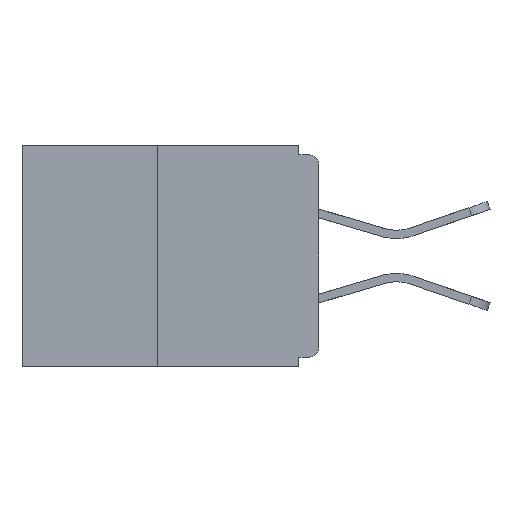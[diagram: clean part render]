
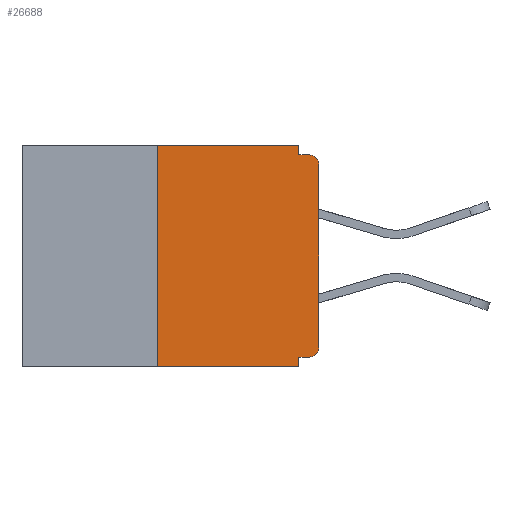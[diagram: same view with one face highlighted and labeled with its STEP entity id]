
A CAD part, left-side view. The second image highlights one B-rep face of the part: STEP entity #26688.
In plain terms, the highlighted planar face has unit normal (-1, 0, 0).
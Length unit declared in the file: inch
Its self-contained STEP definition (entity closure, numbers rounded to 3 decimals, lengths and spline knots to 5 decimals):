
#182 = CARTESIAN_POINT ( 'NONE',  ( 0., 0.031, 0. ) ) ;
#432 = CARTESIAN_POINT ( 'NONE',  ( 0., 0., -0.03 ) ) ;
#718 = VECTOR ( 'NONE', #28998, 39.37008 ) ;
#874 = CARTESIAN_POINT ( 'NONE',  ( 0., 0.031, -0.343 ) ) ;
#924 = DIRECTION ( 'NONE',  ( 1., 0., 0. ) ) ;
#1864 = VERTEX_POINT ( 'NONE', #21137 ) ;
#2328 = ORIENTED_EDGE ( 'NONE', *, *, #19186, .T. ) ;
#2341 = EDGE_CURVE ( 'NONE', #22695, #10764, #21661, .T. ) ;
#2389 = EDGE_LOOP ( 'NONE', ( #16454, #28490, #7199, #27091, #4894, #2328, #24212, #11146, #4104, #2781 ) ) ;
#2548 = DIRECTION ( 'NONE',  ( 0., -1., 0. ) ) ;
#2781 = ORIENTED_EDGE ( 'NONE', *, *, #2341, .F. ) ;
#2846 = CARTESIAN_POINT ( 'NONE',  ( 0., 0., -0.328 ) ) ;
#2960 = EDGE_CURVE ( 'NONE', #22089, #11140, #11749, .T. ) ;
#3183 = DIRECTION ( 'NONE',  ( 0., 0., -1. ) ) ;
#3487 = LINE ( 'NONE', #2846, #718 ) ;
#4104 = ORIENTED_EDGE ( 'NONE', *, *, #16299, .F. ) ;
#4231 = LINE ( 'NONE', #16019, #21391 ) ;
#4462 = AXIS2_PLACEMENT_3D ( 'NONE', #14657, #26265, #18916 ) ;
#4894 = ORIENTED_EDGE ( 'NONE', *, *, #9586, .F. ) ;
#6100 = DIRECTION ( 'NONE',  ( 0., 0., -1. ) ) ;
#6287 = CARTESIAN_POINT ( 'NONE',  ( 0., 0.46, 0. ) ) ;
#6521 = DIRECTION ( 'NONE',  ( 0., 0., 1. ) ) ;
#6545 = LINE ( 'NONE', #10493, #23635 ) ;
#6589 = CARTESIAN_POINT ( 'NONE',  ( 0., 0.46, -0.343 ) ) ;
#7199 = ORIENTED_EDGE ( 'NONE', *, *, #21327, .T. ) ;
#8883 = DIRECTION ( 'NONE',  ( 0., 0., -1. ) ) ;
#9586 = EDGE_CURVE ( 'NONE', #16956, #14985, #3487, .T. ) ;
#9768 = EDGE_CURVE ( 'NONE', #10097, #1864, #6545, .T. ) ;
#10097 = VERTEX_POINT ( 'NONE', #26069 ) ;
#10493 = CARTESIAN_POINT ( 'NONE',  ( 0., 0.25, 0. ) ) ;
#10764 = VERTEX_POINT ( 'NONE', #20231 ) ;
#11140 = VERTEX_POINT ( 'NONE', #432 ) ;
#11146 = ORIENTED_EDGE ( 'NONE', *, *, #27643, .T. ) ;
#11719 = VERTEX_POINT ( 'NONE', #24113 ) ;
#11749 = LINE ( 'NONE', #27129, #12750 ) ;
#11895 = LINE ( 'NONE', #25942, #18970 ) ;
#12056 = VERTEX_POINT ( 'NONE', #12471 ) ;
#12471 = CARTESIAN_POINT ( 'NONE',  ( 0., 0.015, -0.015 ) ) ;
#12750 = VECTOR ( 'NONE', #6521, 39.37008 ) ;
#13713 = AXIS2_PLACEMENT_3D ( 'NONE', #6287, #924, #15182 ) ;
#14065 = DIRECTION ( 'NONE',  ( 0., -1., 0. ) ) ;
#14657 = CARTESIAN_POINT ( 'NONE',  ( 0., 0.015, -0.03 ) ) ;
#14985 = VERTEX_POINT ( 'NONE', #28916 ) ;
#15182 = DIRECTION ( 'NONE',  ( 0., 0., -1. ) ) ;
#15641 = CARTESIAN_POINT ( 'NONE',  ( 0., 0.015, -0.328 ) ) ;
#16019 = CARTESIAN_POINT ( 'NONE',  ( 0., 0., -0.015 ) ) ;
#16299 = EDGE_CURVE ( 'NONE', #10764, #12056, #4231, .T. ) ;
#16454 = ORIENTED_EDGE ( 'NONE', *, *, #21848, .F. ) ;
#16956 = VERTEX_POINT ( 'NONE', #15641 ) ;
#17069 = VECTOR ( 'NONE', #6100, 39.37008 ) ;
#17446 = CARTESIAN_POINT ( 'NONE',  ( 0., 0.015, -0.313 ) ) ;
#18916 = DIRECTION ( 'NONE',  ( 0., 0., -1. ) ) ;
#18970 = VECTOR ( 'NONE', #2548, 39.37008 ) ;
#19078 = CIRCLE ( 'NONE', #4462, 0.015 ) ;
#19186 = EDGE_CURVE ( 'NONE', #16956, #22089, #26212, .T. ) ;
#19540 = LINE ( 'NONE', #874, #22490 ) ;
#20055 = FACE_OUTER_BOUND ( 'NONE', #2389, .T. ) ;
#20231 = CARTESIAN_POINT ( 'NONE',  ( 0., 0.031, -0.015 ) ) ;
#21137 = CARTESIAN_POINT ( 'NONE',  ( 0., 0.25, 0. ) ) ;
#21327 = EDGE_CURVE ( 'NONE', #10097, #11719, #29828, .T. ) ;
#21391 = VECTOR ( 'NONE', #22876, 39.37008 ) ;
#21661 = LINE ( 'NONE', #29165, #17069 ) ;
#21848 = EDGE_CURVE ( 'NONE', #1864, #22695, #11895, .T. ) ;
#22089 = VERTEX_POINT ( 'NONE', #30042 ) ;
#22490 = VECTOR ( 'NONE', #3183, 39.37008 ) ;
#22695 = VERTEX_POINT ( 'NONE', #182 ) ;
#22876 = DIRECTION ( 'NONE',  ( 0., -1., 0. ) ) ;
#23635 = VECTOR ( 'NONE', #29615, 39.37008 ) ;
#24113 = CARTESIAN_POINT ( 'NONE',  ( 0., 0.031, -0.343 ) ) ;
#24212 = ORIENTED_EDGE ( 'NONE', *, *, #2960, .T. ) ;
#24498 = PLANE ( 'NONE',  #13713 ) ;
#24749 = AXIS2_PLACEMENT_3D ( 'NONE', #17446, #26751, #8883 ) ;
#25942 = CARTESIAN_POINT ( 'NONE',  ( 0., 0.46, 0. ) ) ;
#26069 = CARTESIAN_POINT ( 'NONE',  ( 0., 0.25, -0.343 ) ) ;
#26212 = CIRCLE ( 'NONE', #24749, 0.015 ) ;
#26265 = DIRECTION ( 'NONE',  ( -1., 0., 0. ) ) ;
#26688 = ADVANCED_FACE ( 'NONE', ( #20055 ), #24498, .F. ) ;
#26751 = DIRECTION ( 'NONE',  ( -1., 0., 0. ) ) ;
#27091 = ORIENTED_EDGE ( 'NONE', *, *, #28978, .F. ) ;
#27129 = CARTESIAN_POINT ( 'NONE',  ( 0., 0., 0. ) ) ;
#27643 = EDGE_CURVE ( 'NONE', #11140, #12056, #19078, .T. ) ;
#28490 = ORIENTED_EDGE ( 'NONE', *, *, #9768, .F. ) ;
#28916 = CARTESIAN_POINT ( 'NONE',  ( 0., 0.031, -0.328 ) ) ;
#28978 = EDGE_CURVE ( 'NONE', #14985, #11719, #19540, .T. ) ;
#28998 = DIRECTION ( 'NONE',  ( 0., 1., 0. ) ) ;
#29165 = CARTESIAN_POINT ( 'NONE',  ( 0., 0.031, 0. ) ) ;
#29223 = VECTOR ( 'NONE', #14065, 39.37008 ) ;
#29615 = DIRECTION ( 'NONE',  ( 0., 0., 1. ) ) ;
#29828 = LINE ( 'NONE', #6589, #29223 ) ;
#30042 = CARTESIAN_POINT ( 'NONE',  ( 0., 0., -0.313 ) ) ;
